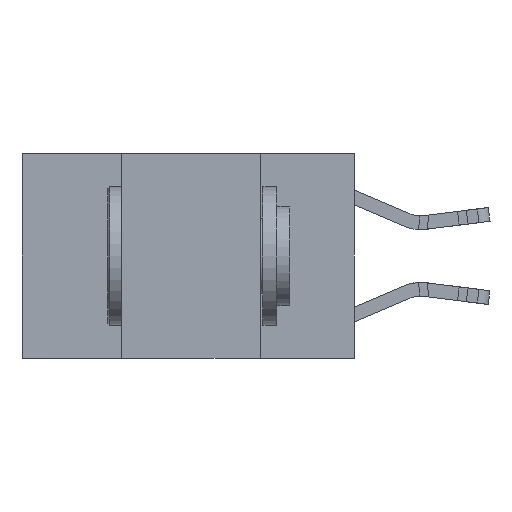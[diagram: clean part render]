
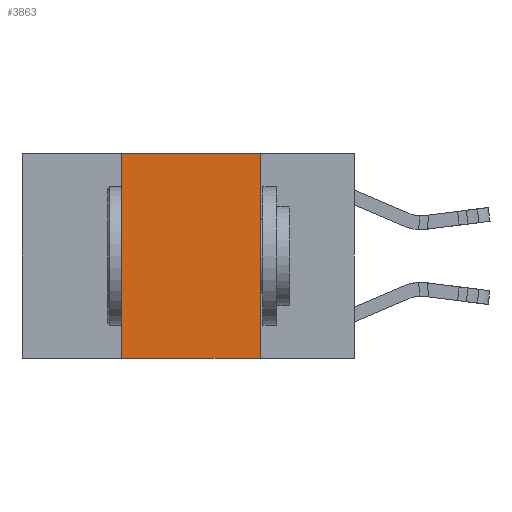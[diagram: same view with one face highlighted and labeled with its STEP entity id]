
A CAD part, left-side view. The second image highlights one B-rep face of the part: STEP entity #3863.
In plain terms, the highlighted planar face has unit normal (-1, 0, 0).
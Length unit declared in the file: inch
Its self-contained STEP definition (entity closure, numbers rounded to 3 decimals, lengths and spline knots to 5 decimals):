
#358 = VERTEX_POINT ( 'NONE', #1241 ) ;
#774 = CARTESIAN_POINT ( 'NONE',  ( 0., 0.42, -0.37 ) ) ;
#1241 = CARTESIAN_POINT ( 'NONE',  ( 0., 0.42, 0. ) ) ;
#2263 = ORIENTED_EDGE ( 'NONE', *, *, #24238, .T. ) ;
#3173 = CARTESIAN_POINT ( 'NONE',  ( 0., 0.42, 0. ) ) ;
#3322 = VECTOR ( 'NONE', #29712, 39.37008 ) ;
#3863 = ADVANCED_FACE ( 'NONE', ( #19390 ), #4585, .F. ) ;
#3964 = AXIS2_PLACEMENT_3D ( 'NONE', #19147, #21522, #7141 ) ;
#4585 = PLANE ( 'NONE',  #3964 ) ;
#4928 = CARTESIAN_POINT ( 'NONE',  ( 0., 0.6, -0.37 ) ) ;
#5690 = CARTESIAN_POINT ( 'NONE',  ( 0., 0.17, 0. ) ) ;
#5970 = CARTESIAN_POINT ( 'NONE',  ( 0., 0.17, -0.37 ) ) ;
#7141 = DIRECTION ( 'NONE',  ( 0., 0., -1. ) ) ;
#7636 = VERTEX_POINT ( 'NONE', #774 ) ;
#8158 = LINE ( 'NONE', #26883, #20178 ) ;
#8853 = EDGE_CURVE ( 'NONE', #7636, #358, #10087, .T. ) ;
#9812 = LINE ( 'NONE', #5690, #3322 ) ;
#10087 = LINE ( 'NONE', #3173, #22082 ) ;
#15516 = EDGE_CURVE ( 'NONE', #22704, #16112, #9812, .T. ) ;
#16112 = VERTEX_POINT ( 'NONE', #5970 ) ;
#16182 = ORIENTED_EDGE ( 'NONE', *, *, #17354, .F. ) ;
#16966 = ORIENTED_EDGE ( 'NONE', *, *, #8853, .F. ) ;
#17067 = DIRECTION ( 'NONE',  ( 0., -1., 0. ) ) ;
#17354 = EDGE_CURVE ( 'NONE', #358, #22704, #8158, .T. ) ;
#17656 = DIRECTION ( 'NONE',  ( 0., 0., 1. ) ) ;
#18446 = VECTOR ( 'NONE', #17067, 39.37008 ) ;
#19147 = CARTESIAN_POINT ( 'NONE',  ( 0., 0.6, 0. ) ) ;
#19390 = FACE_OUTER_BOUND ( 'NONE', #29018, .T. ) ;
#20178 = VECTOR ( 'NONE', #29275, 39.37008 ) ;
#21453 = ORIENTED_EDGE ( 'NONE', *, *, #15516, .F. ) ;
#21522 = DIRECTION ( 'NONE',  ( 1., 0., 0. ) ) ;
#22082 = VECTOR ( 'NONE', #17656, 39.37008 ) ;
#22704 = VERTEX_POINT ( 'NONE', #25500 ) ;
#24238 = EDGE_CURVE ( 'NONE', #7636, #16112, #24786, .T. ) ;
#24786 = LINE ( 'NONE', #4928, #18446 ) ;
#25500 = CARTESIAN_POINT ( 'NONE',  ( 0., 0.17, 0. ) ) ;
#26883 = CARTESIAN_POINT ( 'NONE',  ( 0., 0.6, 0. ) ) ;
#29018 = EDGE_LOOP ( 'NONE', ( #21453, #16182, #16966, #2263 ) ) ;
#29275 = DIRECTION ( 'NONE',  ( 0., -1., 0. ) ) ;
#29712 = DIRECTION ( 'NONE',  ( 0., 0., -1. ) ) ;
